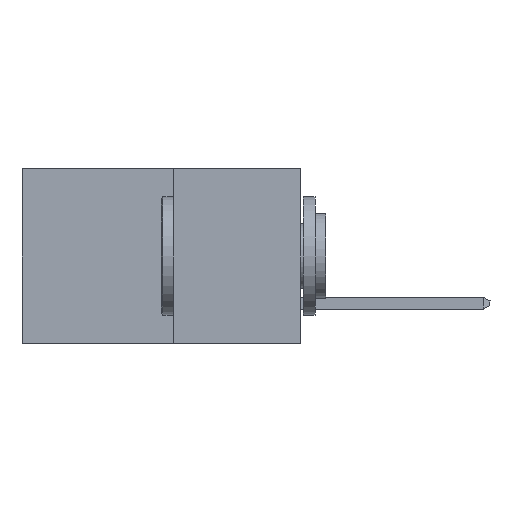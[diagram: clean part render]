
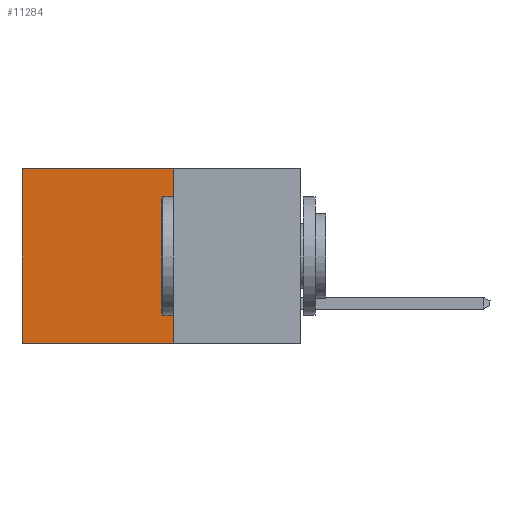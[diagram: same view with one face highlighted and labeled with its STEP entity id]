
A CAD part, left-side view. The second image highlights one B-rep face of the part: STEP entity #11284.
In plain terms, the highlighted planar face has unit normal (-1, 0, 0).
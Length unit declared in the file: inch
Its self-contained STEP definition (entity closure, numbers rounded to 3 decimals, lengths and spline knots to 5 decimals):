
#63 = CARTESIAN_POINT ( 'NONE',  ( 0.277, 0.27, 0. ) ) ;
#610 = EDGE_CURVE ( 'NONE', #8142, #2448, #1091, .T. ) ;
#632 = EDGE_CURVE ( 'NONE', #2448, #8828, #6223, .T. ) ;
#1072 = DIRECTION ( 'NONE',  ( 1., 0., 0. ) ) ;
#1091 = LINE ( 'NONE', #1264, #3928 ) ;
#1264 = CARTESIAN_POINT ( 'NONE',  ( 0.277, 0.27, 0. ) ) ;
#1789 = CARTESIAN_POINT ( 'NONE',  ( 0.277, 0.27, -0.37 ) ) ;
#1986 = CARTESIAN_POINT ( 'NONE',  ( 0.277, 0.59, -0.37 ) ) ;
#2100 = EDGE_CURVE ( 'NONE', #4373, #8828, #4933, .T. ) ;
#2243 = VECTOR ( 'NONE', #7928, 39.37008 ) ;
#2448 = VERTEX_POINT ( 'NONE', #12051 ) ;
#3528 = VECTOR ( 'NONE', #5348, 39.37008 ) ;
#3616 = VECTOR ( 'NONE', #11079, 39.37008 ) ;
#3706 = ORIENTED_EDGE ( 'NONE', *, *, #2100, .F. ) ;
#3928 = VECTOR ( 'NONE', #9142, 39.37008 ) ;
#4373 = VERTEX_POINT ( 'NONE', #13045 ) ;
#4645 = ORIENTED_EDGE ( 'NONE', *, *, #9006, .F. ) ;
#4933 = LINE ( 'NONE', #1789, #2243 ) ;
#5348 = DIRECTION ( 'NONE',  ( 0., 0., -1. ) ) ;
#5904 = ORIENTED_EDGE ( 'NONE', *, *, #632, .T. ) ;
#6223 = LINE ( 'NONE', #8240, #3616 ) ;
#6433 = FACE_OUTER_BOUND ( 'NONE', #9747, .T. ) ;
#7065 = ORIENTED_EDGE ( 'NONE', *, *, #610, .T. ) ;
#7211 = CARTESIAN_POINT ( 'NONE',  ( 0.277, 0.27, -0.37 ) ) ;
#7928 = DIRECTION ( 'NONE',  ( 0., 1., 0. ) ) ;
#8142 = VERTEX_POINT ( 'NONE', #63 ) ;
#8208 = DIRECTION ( 'NONE',  ( 0., 0., -1. ) ) ;
#8240 = CARTESIAN_POINT ( 'NONE',  ( 0.277, 0.59, -0.37 ) ) ;
#8800 = LINE ( 'NONE', #11303, #3528 ) ;
#8828 = VERTEX_POINT ( 'NONE', #1986 ) ;
#9006 = EDGE_CURVE ( 'NONE', #8142, #4373, #8800, .T. ) ;
#9142 = DIRECTION ( 'NONE',  ( 0., 1., 0. ) ) ;
#9747 = EDGE_LOOP ( 'NONE', ( #5904, #3706, #4645, #7065 ) ) ;
#11079 = DIRECTION ( 'NONE',  ( 0., 0., -1. ) ) ;
#11284 = ADVANCED_FACE ( 'NONE', ( #6433 ), #12116, .F. ) ;
#11303 = CARTESIAN_POINT ( 'NONE',  ( 0.277, 0.27, -0.37 ) ) ;
#12051 = CARTESIAN_POINT ( 'NONE',  ( 0.277, 0.59, 0. ) ) ;
#12091 = AXIS2_PLACEMENT_3D ( 'NONE', #7211, #1072, #8208 ) ;
#12116 = PLANE ( 'NONE',  #12091 ) ;
#13045 = CARTESIAN_POINT ( 'NONE',  ( 0.277, 0.27, -0.37 ) ) ;
